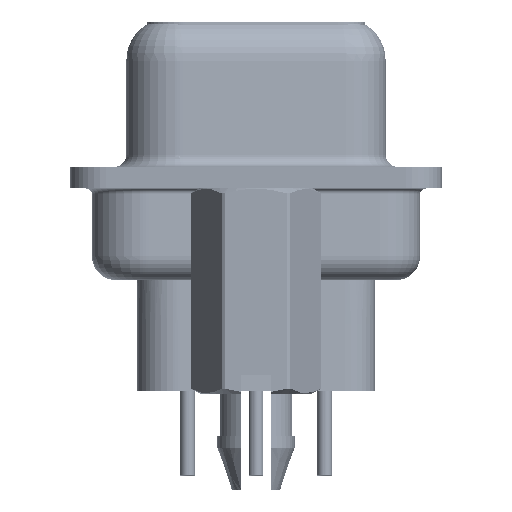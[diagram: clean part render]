
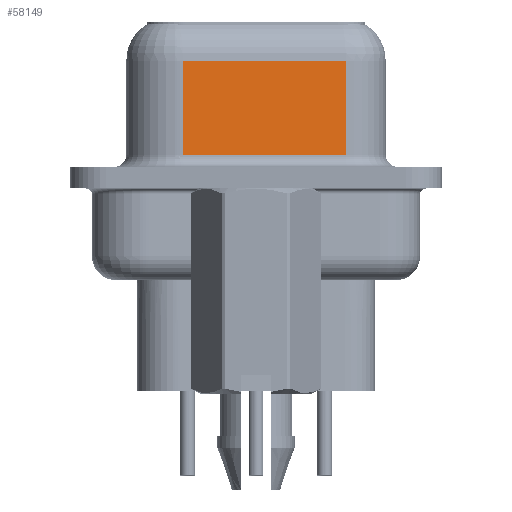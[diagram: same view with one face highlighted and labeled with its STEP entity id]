
A CAD part, left-side view. The second image highlights one B-rep face of the part: STEP entity #58149.
In plain terms, the highlighted planar face has unit normal (-0.985, -0.174, 0).
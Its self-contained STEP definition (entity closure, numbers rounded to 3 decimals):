
#96 = VERTEX_POINT ( 'NONE', #7241 ) ;
#2430 = ORIENTED_EDGE ( 'NONE', *, *, #4824, .F. ) ;
#3404 = EDGE_CURVE ( 'NONE', #19890, #49899, #8041, .T. ) ;
#4824 = EDGE_CURVE ( 'NONE', #19890, #96, #11504, .T. ) ;
#6672 = VECTOR ( 'NONE', #29229, 1000. ) ;
#7241 = CARTESIAN_POINT ( 'NONE',  ( 5.621, -3.722, 0.95 ) ) ;
#8036 = PLANE ( 'NONE',  #28342 ) ;
#8041 = LINE ( 'NONE', #31632, #19048 ) ;
#10428 = LINE ( 'NONE', #34638, #6672 ) ;
#11249 = CARTESIAN_POINT ( 'NONE',  ( 4.43, 3.028, 6.6 ) ) ;
#11504 = LINE ( 'NONE', #50423, #43745 ) ;
#17270 = FACE_OUTER_BOUND ( 'NONE', #30877, .T. ) ;
#17529 = DIRECTION ( 'NONE',  ( 0., 0., -1. ) ) ;
#19048 = VECTOR ( 'NONE', #51116, 1000. ) ;
#19890 = VERTEX_POINT ( 'NONE', #48174 ) ;
#20465 = DIRECTION ( 'NONE',  ( 0., 0., -1. ) ) ;
#22056 = DIRECTION ( 'NONE',  ( -0.174, 0.985, 0. ) ) ;
#22984 = CARTESIAN_POINT ( 'NONE',  ( 5.621, -3.722, 6.6 ) ) ;
#23194 = EDGE_CURVE ( 'NONE', #45005, #96, #10428, .T. ) ;
#25266 = LINE ( 'NONE', #11249, #32617 ) ;
#28342 = AXIS2_PLACEMENT_3D ( 'NONE', #22984, #46932, #22056 ) ;
#29229 = DIRECTION ( 'NONE',  ( 0.174, -0.985, 0. ) ) ;
#30877 = EDGE_LOOP ( 'NONE', ( #2430, #45903, #43681, #61012 ) ) ;
#31632 = CARTESIAN_POINT ( 'NONE',  ( 5.621, -3.722, 4.85 ) ) ;
#32617 = VECTOR ( 'NONE', #20465, 1000. ) ;
#34638 = CARTESIAN_POINT ( 'NONE',  ( 5.621, -3.722, 0.95 ) ) ;
#43681 = ORIENTED_EDGE ( 'NONE', *, *, #44789, .T. ) ;
#43745 = VECTOR ( 'NONE', #17529, 1000. ) ;
#44789 = EDGE_CURVE ( 'NONE', #49899, #45005, #25266, .T. ) ;
#45005 = VERTEX_POINT ( 'NONE', #47872 ) ;
#45903 = ORIENTED_EDGE ( 'NONE', *, *, #3404, .T. ) ;
#46932 = DIRECTION ( 'NONE',  ( 0.985, 0.174, 0. ) ) ;
#47872 = CARTESIAN_POINT ( 'NONE',  ( 4.43, 3.028, 0.95 ) ) ;
#48174 = CARTESIAN_POINT ( 'NONE',  ( 5.621, -3.722, 4.85 ) ) ;
#49899 = VERTEX_POINT ( 'NONE', #59039 ) ;
#50423 = CARTESIAN_POINT ( 'NONE',  ( 5.621, -3.722, 6.6 ) ) ;
#51116 = DIRECTION ( 'NONE',  ( -0.174, 0.985, 0. ) ) ;
#58149 = ADVANCED_FACE ( 'NONE', ( #17270 ), #8036, .F. ) ;
#59039 = CARTESIAN_POINT ( 'NONE',  ( 4.43, 3.028, 4.85 ) ) ;
#61012 = ORIENTED_EDGE ( 'NONE', *, *, #23194, .T. ) ;
